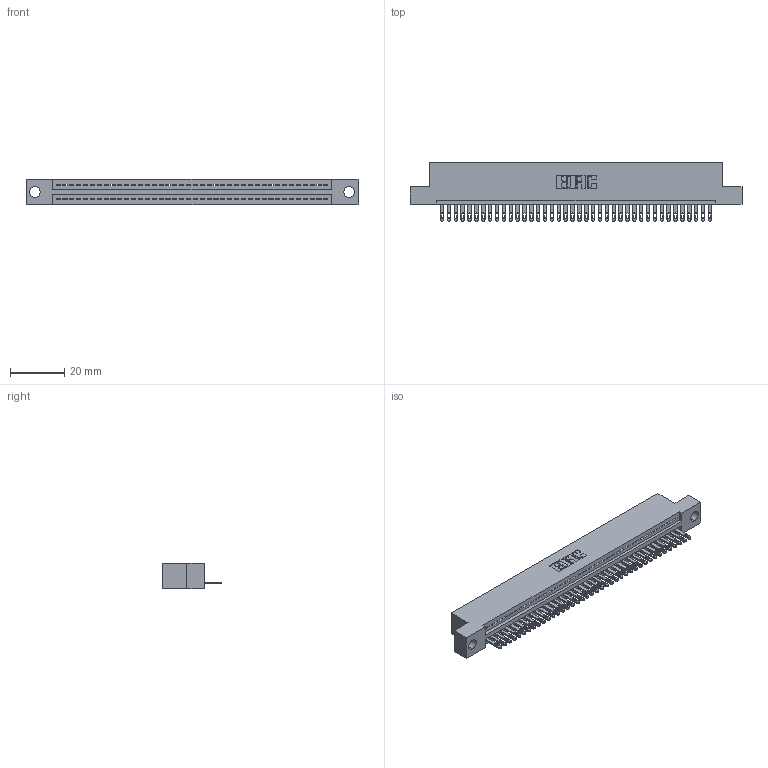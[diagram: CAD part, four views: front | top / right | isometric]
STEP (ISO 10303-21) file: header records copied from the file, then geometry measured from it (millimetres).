
FILE_DESCRIPTION (( 'STEP AP203' ), '1' );
FILE_NAME ('345-040-500-104.STEP', '2018-09-05T00:22:20', ( '' ), ( '' ), 'SwSTEP 2.0', 'SolidWorks 2016', '' );
FILE_SCHEMA (( 'CONFIG_CONTROL_DESIGN' ));
Length unit declared in the file: inch
Products named in the file (3): 345-040-500-104; 345 Part_Flush Mounting Lugs - 0.156 Dia-TH; 345-292-001_345-293-100
Assembly tree (41 placements, depth 2):
  345-040-500-104
    345 Part_Flush Mounting Lugs - 0.156 Dia-TH
    345-292-001_345-293-100  x40
Bounding box: 122.81 x 21.51 x 9.4 mm (x, y, z)
Volume: 11585 mm3; surface area: 15266.9 mm2
Topology: 41 solids, 41 shells, 2286 faces, 7061 edges, 4706 vertices
Faces by surface type: plane 1440, cylinder 846
Entity records: 30307 total; most frequent: CARTESIAN_POINT 5256, ORIENTED_EDGE 5230, DIRECTION 4595, EDGE_CURVE 2615, VECTOR 2319, LINE 2319, VERTEX_POINT 1742, AXIS2_PLACEMENT_3D 1138
